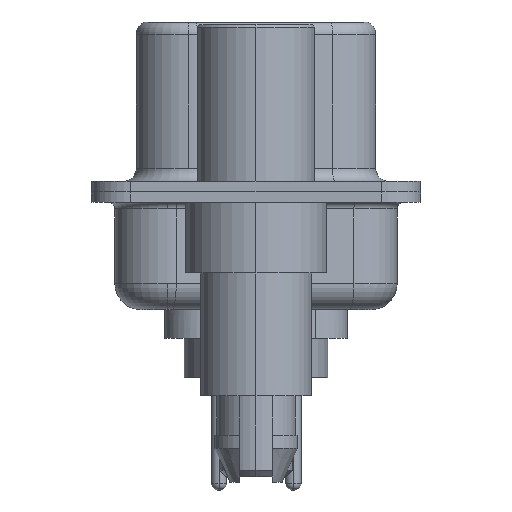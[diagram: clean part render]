
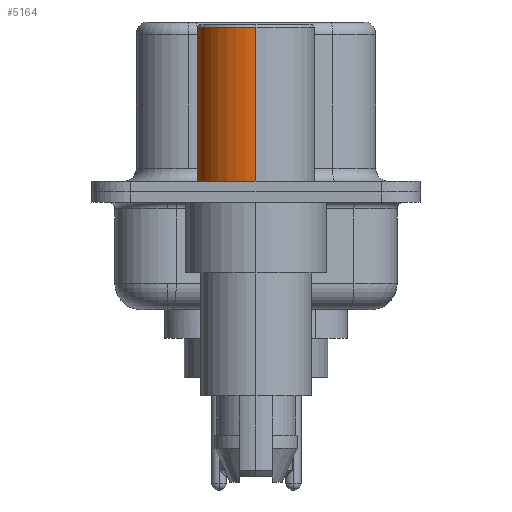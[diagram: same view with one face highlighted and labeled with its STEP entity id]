
A CAD part, left-side view. The second image highlights one B-rep face of the part: STEP entity #5164.
In plain terms, the highlighted cylindrical face has radius 2.25 mm (diameter 4.5 mm), a partial arc.
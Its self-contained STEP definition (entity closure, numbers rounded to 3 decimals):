
#560 = EDGE_LOOP ( 'NONE', ( #18589, #4723, #10270, #15631 ) ) ;
#907 = VERTEX_POINT ( 'NONE', #3454 ) ;
#1148 = CYLINDRICAL_SURFACE ( 'NONE', #3087, 2.25 ) ;
#2127 = DIRECTION ( 'NONE',  ( 0., 0., 1. ) ) ;
#2645 = VERTEX_POINT ( 'NONE', #12362 ) ;
#3087 = AXIS2_PLACEMENT_3D ( 'NONE', #6600, #13898, #8443 ) ;
#3197 = CARTESIAN_POINT ( 'NONE',  ( -2.25, 0., 6.3 ) ) ;
#3454 = CARTESIAN_POINT ( 'NONE',  ( 2.25, 0., 6.3 ) ) ;
#4723 = ORIENTED_EDGE ( 'NONE', *, *, #6181, .T. ) ;
#5164 = ADVANCED_FACE ( 'NONE', ( #10045 ), #1148, .T. ) ;
#6181 = EDGE_CURVE ( 'NONE', #2645, #11998, #19133, .T. ) ;
#6600 = CARTESIAN_POINT ( 'NONE',  ( 0., 0., 0.581 ) ) ;
#7119 = DIRECTION ( 'NONE',  ( 0., 0., 1. ) ) ;
#7273 = AXIS2_PLACEMENT_3D ( 'NONE', #11073, #2127, #12523 ) ;
#7439 = DIRECTION ( 'NONE',  ( 0., 0., 1. ) ) ;
#8190 = EDGE_CURVE ( 'NONE', #18517, #907, #9294, .T. ) ;
#8402 = CARTESIAN_POINT ( 'NONE',  ( -2.25, 0., 0.581 ) ) ;
#8405 = CARTESIAN_POINT ( 'NONE',  ( 2.25, 0., 0.4 ) ) ;
#8443 = DIRECTION ( 'NONE',  ( 1., 0., 0. ) ) ;
#8896 = EDGE_CURVE ( 'NONE', #907, #11998, #18067, .T. ) ;
#9294 = LINE ( 'NONE', #15290, #16444 ) ;
#10045 = FACE_OUTER_BOUND ( 'NONE', #560, .T. ) ;
#10270 = ORIENTED_EDGE ( 'NONE', *, *, #8896, .F. ) ;
#11073 = CARTESIAN_POINT ( 'NONE',  ( 0., 0., 0.4 ) ) ;
#11998 = VERTEX_POINT ( 'NONE', #3197 ) ;
#12362 = CARTESIAN_POINT ( 'NONE',  ( -2.25, 0., 0.4 ) ) ;
#12523 = DIRECTION ( 'NONE',  ( 1., 0., 0. ) ) ;
#13898 = DIRECTION ( 'NONE',  ( 0., 0., 1. ) ) ;
#15290 = CARTESIAN_POINT ( 'NONE',  ( 2.25, 0., 0.581 ) ) ;
#15631 = ORIENTED_EDGE ( 'NONE', *, *, #8190, .F. ) ;
#15753 = CARTESIAN_POINT ( 'NONE',  ( 0., 0., 6.3 ) ) ;
#16444 = VECTOR ( 'NONE', #16811, 1000. ) ;
#16811 = DIRECTION ( 'NONE',  ( 0., 0., 1. ) ) ;
#17245 = DIRECTION ( 'NONE',  ( 1., 0., 0. ) ) ;
#17268 = EDGE_CURVE ( 'NONE', #18517, #2645, #17795, .T. ) ;
#17795 = CIRCLE ( 'NONE', #7273, 2.25 ) ;
#18067 = CIRCLE ( 'NONE', #18716, 2.25 ) ;
#18164 = VECTOR ( 'NONE', #7439, 1000. ) ;
#18517 = VERTEX_POINT ( 'NONE', #8405 ) ;
#18589 = ORIENTED_EDGE ( 'NONE', *, *, #17268, .T. ) ;
#18716 = AXIS2_PLACEMENT_3D ( 'NONE', #15753, #7119, #17245 ) ;
#19133 = LINE ( 'NONE', #8402, #18164 ) ;
